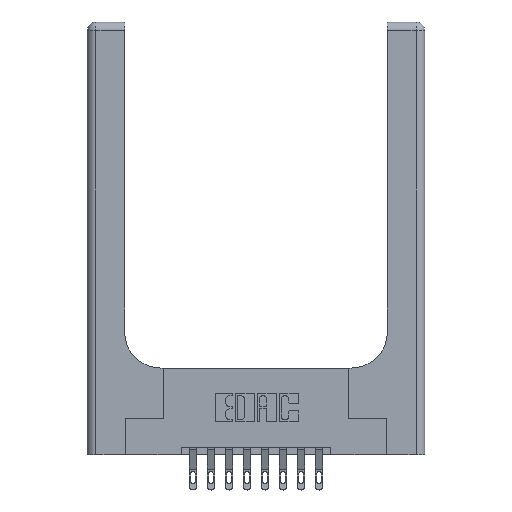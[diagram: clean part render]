
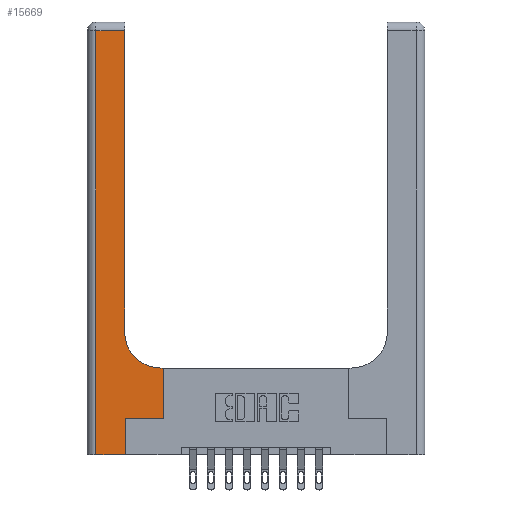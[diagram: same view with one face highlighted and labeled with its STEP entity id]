
A CAD part, top view. The second image highlights one B-rep face of the part: STEP entity #15669.
In plain terms, the highlighted planar face has unit normal (0, 0, 1).
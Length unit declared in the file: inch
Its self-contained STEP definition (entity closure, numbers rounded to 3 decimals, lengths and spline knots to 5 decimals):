
#24 = CARTESIAN_POINT ( 'NONE',  ( 0.26, 0.85, 0.37 ) ) ;
#325 = CARTESIAN_POINT ( 'NONE',  ( 0.06, 0., 0.37 ) ) ;
#498 = ORIENTED_EDGE ( 'NONE', *, *, #8344, .T. ) ;
#526 = CARTESIAN_POINT ( 'NONE',  ( 0., 2.94, 0.37 ) ) ;
#684 = LINE ( 'NONE', #526, #3656 ) ;
#928 = EDGE_CURVE ( 'NONE', #14674, #8338, #8409, .T. ) ;
#1066 = CARTESIAN_POINT ( 'NONE',  ( 0.06, 2.94, 0.37 ) ) ;
#1264 = CARTESIAN_POINT ( 'NONE',  ( 0.528, 0.25, 0.37 ) ) ;
#1596 = CARTESIAN_POINT ( 'NONE',  ( 0.26, 3., 0.37 ) ) ;
#1705 = DIRECTION ( 'NONE',  ( 0., 1., 0. ) ) ;
#1785 = PLANE ( 'NONE',  #9505 ) ;
#1832 = EDGE_LOOP ( 'NONE', ( #3995, #10414, #15416, #2740, #11796, #7956, #498, #14675, #15133 ) ) ;
#1920 = EDGE_CURVE ( 'NONE', #8338, #8336, #12487, .T. ) ;
#2740 = ORIENTED_EDGE ( 'NONE', *, *, #928, .T. ) ;
#2749 = LINE ( 'NONE', #1596, #14906 ) ;
#2857 = DIRECTION ( 'NONE',  ( 0., 0., -1. ) ) ;
#2919 = VECTOR ( 'NONE', #6410, 39.37008 ) ;
#3006 = VECTOR ( 'NONE', #15565, 39.37008 ) ;
#3097 = DIRECTION ( 'NONE',  ( 0., 0., -1. ) ) ;
#3474 = CIRCLE ( 'NONE', #7495, 0.25 ) ;
#3656 = VECTOR ( 'NONE', #12978, 39.37008 ) ;
#3995 = ORIENTED_EDGE ( 'NONE', *, *, #6858, .T. ) ;
#4062 = CARTESIAN_POINT ( 'NONE',  ( 0.51, 0.85, 0.37 ) ) ;
#4280 = VERTEX_POINT ( 'NONE', #14835 ) ;
#4565 = VECTOR ( 'NONE', #14213, 39.37008 ) ;
#4668 = CARTESIAN_POINT ( 'NONE',  ( 0.528, 0.6, 0.37 ) ) ;
#5100 = CARTESIAN_POINT ( 'NONE',  ( 0., 0., 0.37 ) ) ;
#5166 = VERTEX_POINT ( 'NONE', #4668 ) ;
#5199 = EDGE_CURVE ( 'NONE', #5166, #11447, #9598, .T. ) ;
#5258 = CARTESIAN_POINT ( 'NONE',  ( 0.06, 3., 0.37 ) ) ;
#6090 = EDGE_CURVE ( 'NONE', #11447, #13476, #3474, .T. ) ;
#6220 = VERTEX_POINT ( 'NONE', #1066 ) ;
#6317 = CARTESIAN_POINT ( 'NONE',  ( 0.51, 0.6, 0.37 ) ) ;
#6410 = DIRECTION ( 'NONE',  ( 1., 0., 0. ) ) ;
#6597 = VECTOR ( 'NONE', #7123, 39.37008 ) ;
#6656 = CARTESIAN_POINT ( 'NONE',  ( 0., 3., 0.37 ) ) ;
#6858 = EDGE_CURVE ( 'NONE', #13476, #4280, #2749, .T. ) ;
#7123 = DIRECTION ( 'NONE',  ( -1., 0., 0. ) ) ;
#7260 = VERTEX_POINT ( 'NONE', #1264 ) ;
#7495 = AXIS2_PLACEMENT_3D ( 'NONE', #4062, #3097, #11365 ) ;
#7702 = DIRECTION ( 'NONE',  ( -1., 0., 0. ) ) ;
#7956 = ORIENTED_EDGE ( 'NONE', *, *, #15594, .T. ) ;
#8336 = VERTEX_POINT ( 'NONE', #12071 ) ;
#8338 = VERTEX_POINT ( 'NONE', #10536 ) ;
#8344 = EDGE_CURVE ( 'NONE', #7260, #5166, #10776, .T. ) ;
#8409 = LINE ( 'NONE', #5100, #3006 ) ;
#8675 = EDGE_CURVE ( 'NONE', #6220, #14674, #12618, .T. ) ;
#9120 = CARTESIAN_POINT ( 'NONE',  ( 0.265, 0.25, 0.37 ) ) ;
#9505 = AXIS2_PLACEMENT_3D ( 'NONE', #6656, #2857, #7702 ) ;
#9598 = LINE ( 'NONE', #15733, #6597 ) ;
#10078 = CARTESIAN_POINT ( 'NONE',  ( 0.265, 0., 0.37 ) ) ;
#10414 = ORIENTED_EDGE ( 'NONE', *, *, #12458, .T. ) ;
#10536 = CARTESIAN_POINT ( 'NONE',  ( 0.265, 0., 0.37 ) ) ;
#10776 = LINE ( 'NONE', #15640, #4565 ) ;
#11174 = VECTOR ( 'NONE', #1705, 39.37008 ) ;
#11210 = VECTOR ( 'NONE', #15079, 39.37008 ) ;
#11365 = DIRECTION ( 'NONE',  ( 1., 0., 0. ) ) ;
#11447 = VERTEX_POINT ( 'NONE', #6317 ) ;
#11796 = ORIENTED_EDGE ( 'NONE', *, *, #1920, .T. ) ;
#12071 = CARTESIAN_POINT ( 'NONE',  ( 0.265, 0.25, 0.37 ) ) ;
#12458 = EDGE_CURVE ( 'NONE', #4280, #6220, #684, .T. ) ;
#12487 = LINE ( 'NONE', #10078, #11174 ) ;
#12618 = LINE ( 'NONE', #5258, #11210 ) ;
#12978 = DIRECTION ( 'NONE',  ( -1., 0., 0. ) ) ;
#13476 = VERTEX_POINT ( 'NONE', #24 ) ;
#13766 = FACE_OUTER_BOUND ( 'NONE', #1832, .T. ) ;
#13895 = DIRECTION ( 'NONE',  ( 0., 1., 0. ) ) ;
#13998 = LINE ( 'NONE', #9120, #2919 ) ;
#14213 = DIRECTION ( 'NONE',  ( 0., 1., 0. ) ) ;
#14674 = VERTEX_POINT ( 'NONE', #325 ) ;
#14675 = ORIENTED_EDGE ( 'NONE', *, *, #5199, .T. ) ;
#14835 = CARTESIAN_POINT ( 'NONE',  ( 0.26, 2.94, 0.37 ) ) ;
#14906 = VECTOR ( 'NONE', #13895, 39.37008 ) ;
#15079 = DIRECTION ( 'NONE',  ( 0., -1., 0. ) ) ;
#15133 = ORIENTED_EDGE ( 'NONE', *, *, #6090, .T. ) ;
#15416 = ORIENTED_EDGE ( 'NONE', *, *, #8675, .T. ) ;
#15565 = DIRECTION ( 'NONE',  ( 1., 0., 0. ) ) ;
#15594 = EDGE_CURVE ( 'NONE', #8336, #7260, #13998, .T. ) ;
#15640 = CARTESIAN_POINT ( 'NONE',  ( 0.528, 0.25, 0.37 ) ) ;
#15669 = ADVANCED_FACE ( 'NONE', ( #13766 ), #1785, .F. ) ;
#15733 = CARTESIAN_POINT ( 'NONE',  ( 0.26, 0.6, 0.37 ) ) ;
